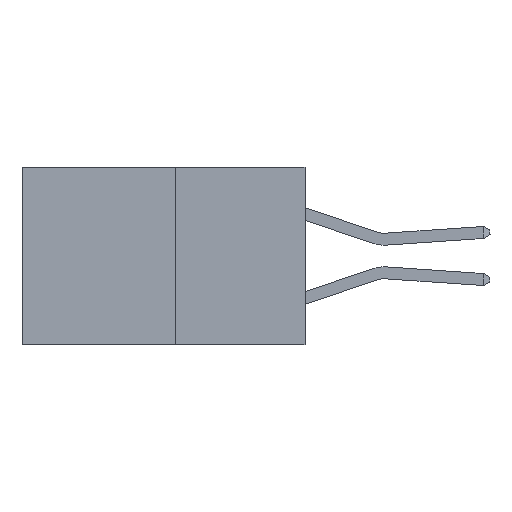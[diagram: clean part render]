
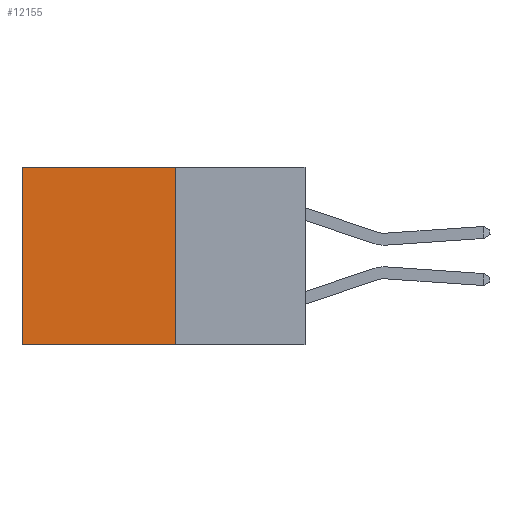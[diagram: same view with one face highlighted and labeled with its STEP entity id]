
A CAD part, left-side view. The second image highlights one B-rep face of the part: STEP entity #12155.
In plain terms, the highlighted planar face has unit normal (-1, 0, 0).
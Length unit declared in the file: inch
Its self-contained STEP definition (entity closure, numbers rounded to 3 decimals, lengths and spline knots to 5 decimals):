
#129 = CARTESIAN_POINT ( 'NONE',  ( 0.277, 0.59, -0.37 ) ) ;
#458 = VERTEX_POINT ( 'NONE', #8902 ) ;
#490 = VECTOR ( 'NONE', #14210, 39.37008 ) ;
#500 = VECTOR ( 'NONE', #3396, 39.37008 ) ;
#1359 = VECTOR ( 'NONE', #10148, 39.37008 ) ;
#1774 = PLANE ( 'NONE',  #10670 ) ;
#2052 = EDGE_CURVE ( 'NONE', #6553, #4741, #14861, .T. ) ;
#3396 = DIRECTION ( 'NONE',  ( 0., 0., -1. ) ) ;
#3863 = ORIENTED_EDGE ( 'NONE', *, *, #13546, .T. ) ;
#4504 = DIRECTION ( 'NONE',  ( 0., 0., -1. ) ) ;
#4741 = VERTEX_POINT ( 'NONE', #6537 ) ;
#5108 = ORIENTED_EDGE ( 'NONE', *, *, #13502, .F. ) ;
#5206 = FACE_OUTER_BOUND ( 'NONE', #12979, .T. ) ;
#5607 = LINE ( 'NONE', #10314, #15064 ) ;
#6130 = CARTESIAN_POINT ( 'NONE',  ( 0.277, 0.59, -0.37 ) ) ;
#6537 = CARTESIAN_POINT ( 'NONE',  ( 0.277, 0.27, -0.37 ) ) ;
#6553 = VERTEX_POINT ( 'NONE', #6884 ) ;
#6884 = CARTESIAN_POINT ( 'NONE',  ( 0.277, 0.27, 0. ) ) ;
#8902 = CARTESIAN_POINT ( 'NONE',  ( 0.277, 0.59, 0. ) ) ;
#9046 = EDGE_CURVE ( 'NONE', #6553, #458, #5607, .T. ) ;
#9886 = ORIENTED_EDGE ( 'NONE', *, *, #9046, .T. ) ;
#10148 = DIRECTION ( 'NONE',  ( 0., 1., 0. ) ) ;
#10314 = CARTESIAN_POINT ( 'NONE',  ( 0.277, 0.27, 0. ) ) ;
#10670 = AXIS2_PLACEMENT_3D ( 'NONE', #13895, #12653, #4504 ) ;
#11464 = VERTEX_POINT ( 'NONE', #129 ) ;
#11763 = ORIENTED_EDGE ( 'NONE', *, *, #2052, .F. ) ;
#12155 = ADVANCED_FACE ( 'NONE', ( #5206 ), #1774, .F. ) ;
#12653 = DIRECTION ( 'NONE',  ( 1., 0., 0. ) ) ;
#12856 = CARTESIAN_POINT ( 'NONE',  ( 0.277, 0.27, -0.37 ) ) ;
#12979 = EDGE_LOOP ( 'NONE', ( #3863, #5108, #11763, #9886 ) ) ;
#13319 = CARTESIAN_POINT ( 'NONE',  ( 0.277, 0.27, -0.37 ) ) ;
#13502 = EDGE_CURVE ( 'NONE', #4741, #11464, #15260, .T. ) ;
#13546 = EDGE_CURVE ( 'NONE', #458, #11464, #14866, .T. ) ;
#13895 = CARTESIAN_POINT ( 'NONE',  ( 0.277, 0.27, -0.37 ) ) ;
#14210 = DIRECTION ( 'NONE',  ( 0., 0., -1. ) ) ;
#14284 = DIRECTION ( 'NONE',  ( 0., 1., 0. ) ) ;
#14861 = LINE ( 'NONE', #13319, #490 ) ;
#14866 = LINE ( 'NONE', #6130, #500 ) ;
#15064 = VECTOR ( 'NONE', #14284, 39.37008 ) ;
#15260 = LINE ( 'NONE', #12856, #1359 ) ;
